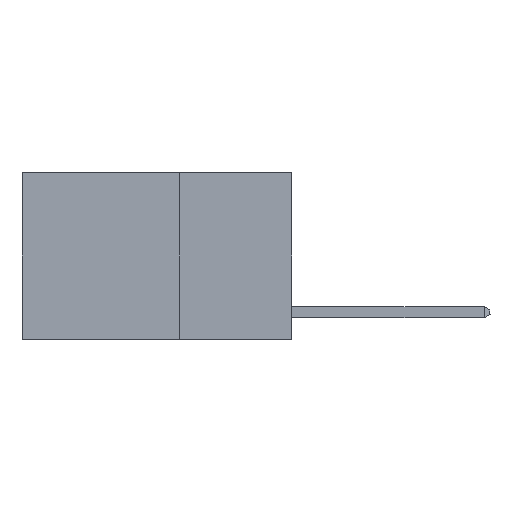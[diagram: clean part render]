
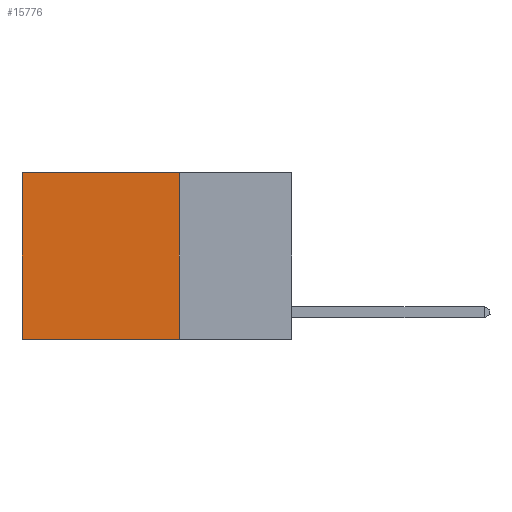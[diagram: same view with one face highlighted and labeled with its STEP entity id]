
A CAD part, left-side view. The second image highlights one B-rep face of the part: STEP entity #15776.
In plain terms, the highlighted planar face has unit normal (-1, 0, 0).
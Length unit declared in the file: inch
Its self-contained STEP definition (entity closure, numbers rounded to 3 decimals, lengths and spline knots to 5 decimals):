
#1536 = CARTESIAN_POINT ( 'NONE',  ( 0.2625, 0.6, -0.37 ) ) ;
#2780 = CARTESIAN_POINT ( 'NONE',  ( 0.2625, 0.25, 0. ) ) ;
#3455 = EDGE_CURVE ( 'NONE', #12521, #24218, #7441, .T. ) ;
#3525 = AXIS2_PLACEMENT_3D ( 'NONE', #3775, #20611, #7631 ) ;
#3775 = CARTESIAN_POINT ( 'NONE',  ( 0.2625, 0.25, 0. ) ) ;
#5457 = ORIENTED_EDGE ( 'NONE', *, *, #24167, .F. ) ;
#5525 = CARTESIAN_POINT ( 'NONE',  ( 0.2625, 0.25, -0.37 ) ) ;
#5526 = VECTOR ( 'NONE', #18895, 39.37008 ) ;
#5793 = VERTEX_POINT ( 'NONE', #1536 ) ;
#6449 = CARTESIAN_POINT ( 'NONE',  ( 0.2625, 0.25, -0.37 ) ) ;
#7441 = LINE ( 'NONE', #2780, #13822 ) ;
#7631 = DIRECTION ( 'NONE',  ( 0., 0., -1. ) ) ;
#8267 = VECTOR ( 'NONE', #18166, 39.37008 ) ;
#9220 = DIRECTION ( 'NONE',  ( 0., 1., 0. ) ) ;
#9553 = FACE_OUTER_BOUND ( 'NONE', #25598, .T. ) ;
#9735 = LINE ( 'NONE', #24341, #14716 ) ;
#9838 = CARTESIAN_POINT ( 'NONE',  ( 0.2625, 0.6, 0. ) ) ;
#10276 = EDGE_CURVE ( 'NONE', #24218, #5793, #17903, .T. ) ;
#10599 = ORIENTED_EDGE ( 'NONE', *, *, #3455, .T. ) ;
#12521 = VERTEX_POINT ( 'NONE', #12791 ) ;
#12791 = CARTESIAN_POINT ( 'NONE',  ( 0.2625, 0.25, 0. ) ) ;
#13822 = VECTOR ( 'NONE', #9220, 39.37008 ) ;
#14716 = VECTOR ( 'NONE', #24086, 39.37008 ) ;
#15776 = ADVANCED_FACE ( 'NONE', ( #9553 ), #26620, .F. ) ;
#15812 = ORIENTED_EDGE ( 'NONE', *, *, #10276, .T. ) ;
#15904 = LINE ( 'NONE', #6449, #5526 ) ;
#17903 = LINE ( 'NONE', #9838, #8267 ) ;
#18166 = DIRECTION ( 'NONE',  ( 0., 0., -1. ) ) ;
#18895 = DIRECTION ( 'NONE',  ( 0., 1., 0. ) ) ;
#20156 = VERTEX_POINT ( 'NONE', #5525 ) ;
#20611 = DIRECTION ( 'NONE',  ( 1., 0., 0. ) ) ;
#24086 = DIRECTION ( 'NONE',  ( 0., 0., -1. ) ) ;
#24167 = EDGE_CURVE ( 'NONE', #20156, #5793, #15904, .T. ) ;
#24218 = VERTEX_POINT ( 'NONE', #24774 ) ;
#24341 = CARTESIAN_POINT ( 'NONE',  ( 0.2625, 0.25, 0. ) ) ;
#24518 = EDGE_CURVE ( 'NONE', #12521, #20156, #9735, .T. ) ;
#24632 = ORIENTED_EDGE ( 'NONE', *, *, #24518, .F. ) ;
#24774 = CARTESIAN_POINT ( 'NONE',  ( 0.2625, 0.6, 0. ) ) ;
#25598 = EDGE_LOOP ( 'NONE', ( #15812, #5457, #24632, #10599 ) ) ;
#26620 = PLANE ( 'NONE',  #3525 ) ;
